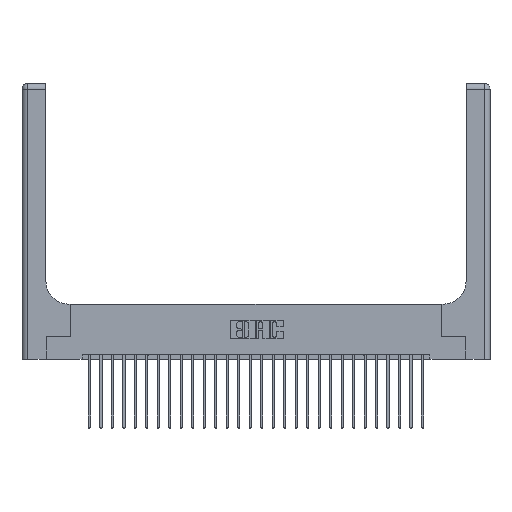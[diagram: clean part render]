
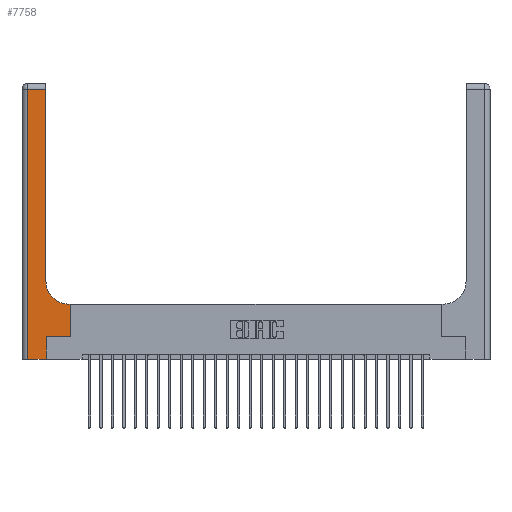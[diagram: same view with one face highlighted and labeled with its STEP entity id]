
A CAD part, top view. The second image highlights one B-rep face of the part: STEP entity #7758.
In plain terms, the highlighted planar face has unit normal (0, 0, 1).
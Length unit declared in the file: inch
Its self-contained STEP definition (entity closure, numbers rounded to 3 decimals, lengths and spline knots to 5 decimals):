
#156 = VECTOR ( 'NONE', #11944, 39.37008 ) ;
#263 = DIRECTION ( 'NONE',  ( 0., 1., 0. ) ) ;
#601 = CARTESIAN_POINT ( 'NONE',  ( 0.06, 0., 0.37 ) ) ;
#1018 = ORIENTED_EDGE ( 'NONE', *, *, #16400, .T. ) ;
#1355 = LINE ( 'NONE', #17931, #3442 ) ;
#1981 = VERTEX_POINT ( 'NONE', #3352 ) ;
#2320 = ORIENTED_EDGE ( 'NONE', *, *, #11983, .T. ) ;
#2407 = EDGE_CURVE ( 'NONE', #3481, #3673, #12516, .T. ) ;
#2776 = PLANE ( 'NONE',  #22855 ) ;
#3352 = CARTESIAN_POINT ( 'NONE',  ( 0.06, 2.94, 0.37 ) ) ;
#3442 = VECTOR ( 'NONE', #263, 39.37008 ) ;
#3445 = DIRECTION ( 'NONE',  ( 1., 0., 0. ) ) ;
#3481 = VERTEX_POINT ( 'NONE', #23771 ) ;
#3612 = CARTESIAN_POINT ( 'NONE',  ( 0.265, 0., 0.37 ) ) ;
#3673 = VERTEX_POINT ( 'NONE', #19742 ) ;
#3772 = CARTESIAN_POINT ( 'NONE',  ( 0., 2.94, 0.37 ) ) ;
#4203 = CARTESIAN_POINT ( 'NONE',  ( 0.26, 3., 0.37 ) ) ;
#5196 = ORIENTED_EDGE ( 'NONE', *, *, #13348, .T. ) ;
#5325 = LINE ( 'NONE', #4203, #10431 ) ;
#5718 = CARTESIAN_POINT ( 'NONE',  ( 0.51, 0.85, 0.37 ) ) ;
#6801 = CARTESIAN_POINT ( 'NONE',  ( 0.528, 0.6, 0.37 ) ) ;
#7276 = LINE ( 'NONE', #21636, #21764 ) ;
#7758 = ADVANCED_FACE ( 'NONE', ( #12990 ), #2776, .F. ) ;
#9504 = CARTESIAN_POINT ( 'NONE',  ( 0.26, 0.6, 0.37 ) ) ;
#9570 = EDGE_CURVE ( 'NONE', #17419, #3481, #13320, .T. ) ;
#9766 = VERTEX_POINT ( 'NONE', #16674 ) ;
#9988 = CARTESIAN_POINT ( 'NONE',  ( 0., 0., 0.37 ) ) ;
#10070 = VECTOR ( 'NONE', #16430, 39.37008 ) ;
#10431 = VECTOR ( 'NONE', #26633, 39.37008 ) ;
#11127 = DIRECTION ( 'NONE',  ( 0., 0., -1. ) ) ;
#11165 = ORIENTED_EDGE ( 'NONE', *, *, #9570, .T. ) ;
#11865 = VERTEX_POINT ( 'NONE', #12708 ) ;
#11944 = DIRECTION ( 'NONE',  ( 0., 1., 0. ) ) ;
#11983 = EDGE_CURVE ( 'NONE', #20634, #11865, #26480, .T. ) ;
#12105 = DIRECTION ( 'NONE',  ( -1., 0., 0. ) ) ;
#12302 = VECTOR ( 'NONE', #3445, 39.37008 ) ;
#12516 = CIRCLE ( 'NONE', #18994, 0.25 ) ;
#12529 = CARTESIAN_POINT ( 'NONE',  ( 0.265, 0.25, 0.37 ) ) ;
#12708 = CARTESIAN_POINT ( 'NONE',  ( 0.528, 0.25, 0.37 ) ) ;
#12990 = FACE_OUTER_BOUND ( 'NONE', #25146, .T. ) ;
#13320 = LINE ( 'NONE', #9504, #14502 ) ;
#13348 = EDGE_CURVE ( 'NONE', #18690, #1981, #22372, .T. ) ;
#14117 = CARTESIAN_POINT ( 'NONE',  ( 0.265, 0.25, 0.37 ) ) ;
#14201 = EDGE_CURVE ( 'NONE', #11865, #17419, #1355, .T. ) ;
#14350 = ORIENTED_EDGE ( 'NONE', *, *, #14201, .T. ) ;
#14502 = VECTOR ( 'NONE', #21569, 39.37008 ) ;
#15165 = ORIENTED_EDGE ( 'NONE', *, *, #2407, .T. ) ;
#15353 = EDGE_CURVE ( 'NONE', #22939, #9766, #21916, .T. ) ;
#16400 = EDGE_CURVE ( 'NONE', #9766, #20634, #22209, .T. ) ;
#16430 = DIRECTION ( 'NONE',  ( 1., 0., 0. ) ) ;
#16451 = CARTESIAN_POINT ( 'NONE',  ( 0.26, 2.94, 0.37 ) ) ;
#16674 = CARTESIAN_POINT ( 'NONE',  ( 0.265, 0., 0.37 ) ) ;
#17166 = CARTESIAN_POINT ( 'NONE',  ( 0., 3., 0.37 ) ) ;
#17419 = VERTEX_POINT ( 'NONE', #6801 ) ;
#17525 = DIRECTION ( 'NONE',  ( 0., 0., -1. ) ) ;
#17931 = CARTESIAN_POINT ( 'NONE',  ( 0.528, 0.25, 0.37 ) ) ;
#18690 = VERTEX_POINT ( 'NONE', #16451 ) ;
#18994 = AXIS2_PLACEMENT_3D ( 'NONE', #5718, #17525, #23758 ) ;
#19336 = DIRECTION ( 'NONE',  ( -1., 0., 0. ) ) ;
#19742 = CARTESIAN_POINT ( 'NONE',  ( 0.26, 0.85, 0.37 ) ) ;
#20614 = EDGE_CURVE ( 'NONE', #3673, #18690, #5325, .T. ) ;
#20634 = VERTEX_POINT ( 'NONE', #12529 ) ;
#21130 = ORIENTED_EDGE ( 'NONE', *, *, #20614, .T. ) ;
#21569 = DIRECTION ( 'NONE',  ( -1., 0., 0. ) ) ;
#21636 = CARTESIAN_POINT ( 'NONE',  ( 0.06, 3., 0.37 ) ) ;
#21764 = VECTOR ( 'NONE', #21902, 39.37008 ) ;
#21902 = DIRECTION ( 'NONE',  ( 0., -1., 0. ) ) ;
#21916 = LINE ( 'NONE', #9988, #12302 ) ;
#22209 = LINE ( 'NONE', #3612, #156 ) ;
#22372 = LINE ( 'NONE', #3772, #25076 ) ;
#22855 = AXIS2_PLACEMENT_3D ( 'NONE', #17166, #11127, #19336 ) ;
#22939 = VERTEX_POINT ( 'NONE', #601 ) ;
#22959 = ORIENTED_EDGE ( 'NONE', *, *, #26076, .T. ) ;
#23758 = DIRECTION ( 'NONE',  ( 1., 0., 0. ) ) ;
#23771 = CARTESIAN_POINT ( 'NONE',  ( 0.51, 0.6, 0.37 ) ) ;
#24477 = ORIENTED_EDGE ( 'NONE', *, *, #15353, .T. ) ;
#25076 = VECTOR ( 'NONE', #12105, 39.37008 ) ;
#25146 = EDGE_LOOP ( 'NONE', ( #21130, #5196, #22959, #24477, #1018, #2320, #14350, #11165, #15165 ) ) ;
#26076 = EDGE_CURVE ( 'NONE', #1981, #22939, #7276, .T. ) ;
#26480 = LINE ( 'NONE', #14117, #10070 ) ;
#26633 = DIRECTION ( 'NONE',  ( 0., 1., 0. ) ) ;
